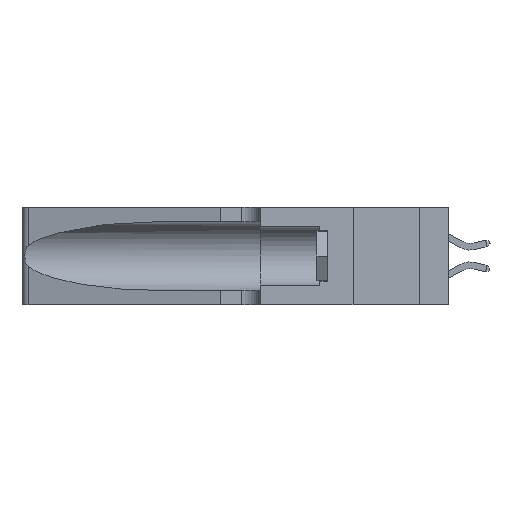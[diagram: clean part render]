
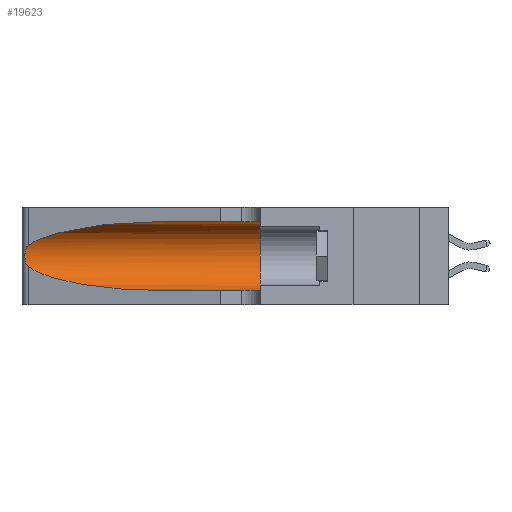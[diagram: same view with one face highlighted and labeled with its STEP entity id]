
A CAD part, left-side view. The second image highlights one B-rep face of the part: STEP entity #19623.
In plain terms, the highlighted cylindrical face has radius 3.308 mm (diameter 6.617 mm), a partial arc.
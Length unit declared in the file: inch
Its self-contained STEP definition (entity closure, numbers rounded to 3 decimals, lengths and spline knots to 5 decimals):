
#348 = EDGE_CURVE ( 'NONE', #20561, #9928, #9784, .T. ) ;
#477 = VERTEX_POINT ( 'NONE', #13632 ) ;
#497 = CARTESIAN_POINT ( 'NONE',  ( 0.25639, 1.23184, 0.21858 ) ) ;
#596 = DIRECTION ( 'NONE',  ( 0., 0., -1. ) ) ;
#694 = CARTESIAN_POINT ( 'NONE',  ( 0.1305, 0.72297, 0.31525 ) ) ;
#824 = CARTESIAN_POINT ( 'NONE',  ( 0.18966, 0.96281, 0.31525 ) ) ;
#1361 = CARTESIAN_POINT ( 'NONE',  ( 0.1305, 0.72297, 0.05475 ) ) ;
#1520 = CARTESIAN_POINT ( 'NONE',  ( 0.1305, 0.35, 0.05475 ) ) ;
#2295 = CARTESIAN_POINT ( 'NONE',  ( 0.25854, 1.2359, 0.20912 ) ) ;
#2627 = CARTESIAN_POINT ( 'NONE',  ( 0.25487, 1.22718, 0.22369 ) ) ;
#2649 =( BOUNDED_CURVE ( )  B_SPLINE_CURVE ( 3, ( #12767, #824, #5948, #2627 ),
 .UNSPECIFIED., .F., .F. ) 
 B_SPLINE_CURVE_WITH_KNOTS ( ( 4, 4 ),
 ( 1.5708, 2.84003 ),
 .UNSPECIFIED. ) 
 CURVE ( )  GEOMETRIC_REPRESENTATION_ITEM ( )  RATIONAL_B_SPLINE_CURVE ( ( 1., 0.87, 0.87, 1. ) ) 
 REPRESENTATION_ITEM ( '' )  );
#2692 = EDGE_CURVE ( 'NONE', #17961, #15681, #2649, .T. ) ;
#4013 = CARTESIAN_POINT ( 'NONE',  ( 0.26075, 1.23896, 0.19203 ) ) ;
#4035 = CARTESIAN_POINT ( 'NONE',  ( 0.25487, 1.22718, 0.14631 ) ) ;
#4983 =( BOUNDED_CURVE ( )  B_SPLINE_CURVE ( 3, ( #10450, #20434, #18830, #8816 ),
 .UNSPECIFIED., .F., .F. ) 
 B_SPLINE_CURVE_WITH_KNOTS ( ( 4, 4 ),
 ( 3.44316, 4.71239 ),
 .UNSPECIFIED. ) 
 CURVE ( )  GEOMETRIC_REPRESENTATION_ITEM ( )  RATIONAL_B_SPLINE_CURVE ( ( 1., 0.87, 0.87, 1. ) ) 
 REPRESENTATION_ITEM ( '' )  );
#5169 = CARTESIAN_POINT ( 'NONE',  ( 0.1305, 1.61858, 0.185 ) ) ;
#5713 = CARTESIAN_POINT ( 'NONE',  ( 0.26017, 1.23833, 0.17102 ) ) ;
#5948 = CARTESIAN_POINT ( 'NONE',  ( 0.2373, 1.15595, 0.28018 ) ) ;
#6148 = ORIENTED_EDGE ( 'NONE', *, *, #12229, .T. ) ;
#6439 = B_SPLINE_CURVE_WITH_KNOTS ( 'NONE', 3,
 ( #7318, #8997, #497, #12452, #2295, #14146, #4013, #15793, #5713, #17450, #7391, #19094, #9061, #20764 ),
 .UNSPECIFIED., .F., .F.,
 ( 4, 2, 2, 2, 2, 2, 4 ),
 ( 0., 0.00027, 0.00053, 0.00107, 0.0016, 0.00187, 0.00214 ),
 .UNSPECIFIED. ) ;
#7070 = DIRECTION ( 'NONE',  ( 0., -1., 0. ) ) ;
#7318 = CARTESIAN_POINT ( 'NONE',  ( 0.25487, 1.22718, 0.22369 ) ) ;
#7391 = CARTESIAN_POINT ( 'NONE',  ( 0.25789, 1.23486, 0.15765 ) ) ;
#7710 = LINE ( 'NONE', #12209, #19467 ) ;
#8169 = CIRCLE ( 'NONE', #14842, 0.13025 ) ;
#8256 = AXIS2_PLACEMENT_3D ( 'NONE', #5169, #10254, #596 ) ;
#8816 = CARTESIAN_POINT ( 'NONE',  ( 0.1305, 0.72297, 0.05475 ) ) ;
#8997 = CARTESIAN_POINT ( 'NONE',  ( 0.25555, 1.22994, 0.2215 ) ) ;
#9061 = CARTESIAN_POINT ( 'NONE',  ( 0.25555, 1.22993, 0.14849 ) ) ;
#9579 = VERTEX_POINT ( 'NONE', #4035 ) ;
#9784 = LINE ( 'NONE', #16242, #18178 ) ;
#9842 = DIRECTION ( 'NONE',  ( 0., 1., 0. ) ) ;
#9928 = VERTEX_POINT ( 'NONE', #1520 ) ;
#10254 = DIRECTION ( 'NONE',  ( 0., -1., 0. ) ) ;
#10450 = CARTESIAN_POINT ( 'NONE',  ( 0.25487, 1.22718, 0.14631 ) ) ;
#12209 = CARTESIAN_POINT ( 'NONE',  ( 0.1305, 1.61858, 0.31525 ) ) ;
#12229 = EDGE_CURVE ( 'NONE', #15681, #9579, #6439, .T. ) ;
#12452 = CARTESIAN_POINT ( 'NONE',  ( 0.25787, 1.23484, 0.2124 ) ) ;
#12767 = CARTESIAN_POINT ( 'NONE',  ( 0.1305, 0.72297, 0.31525 ) ) ;
#13197 = EDGE_CURVE ( 'NONE', #477, #9928, #8169, .T. ) ;
#13479 = FACE_OUTER_BOUND ( 'NONE', #16182, .T. ) ;
#13497 = EDGE_CURVE ( 'NONE', #9579, #20561, #4983, .T. ) ;
#13632 = CARTESIAN_POINT ( 'NONE',  ( 0.1305, 0.35, 0.31525 ) ) ;
#14146 = CARTESIAN_POINT ( 'NONE',  ( 0.26018, 1.23835, 0.19895 ) ) ;
#14842 = AXIS2_PLACEMENT_3D ( 'NONE', #19849, #9842, #21498 ) ;
#15394 = ORIENTED_EDGE ( 'NONE', *, *, #13197, .F. ) ;
#15681 = VERTEX_POINT ( 'NONE', #20165 ) ;
#15793 = CARTESIAN_POINT ( 'NONE',  ( 0.26075, 1.23896, 0.178 ) ) ;
#16182 = EDGE_LOOP ( 'NONE', ( #18990, #6148, #19497, #16521, #15394, #21078 ) ) ;
#16242 = CARTESIAN_POINT ( 'NONE',  ( 0.1305, 1.61858, 0.05475 ) ) ;
#16521 = ORIENTED_EDGE ( 'NONE', *, *, #348, .T. ) ;
#17204 = DIRECTION ( 'NONE',  ( 0., -1., 0. ) ) ;
#17450 = CARTESIAN_POINT ( 'NONE',  ( 0.25856, 1.23593, 0.16098 ) ) ;
#17784 = EDGE_CURVE ( 'NONE', #17961, #477, #7710, .T. ) ;
#17961 = VERTEX_POINT ( 'NONE', #694 ) ;
#18178 = VECTOR ( 'NONE', #17204, 39.37008 ) ;
#18830 = CARTESIAN_POINT ( 'NONE',  ( 0.18966, 0.96281, 0.05475 ) ) ;
#18990 = ORIENTED_EDGE ( 'NONE', *, *, #2692, .T. ) ;
#19094 = CARTESIAN_POINT ( 'NONE',  ( 0.25639, 1.23186, 0.15144 ) ) ;
#19467 = VECTOR ( 'NONE', #7070, 39.37008 ) ;
#19497 = ORIENTED_EDGE ( 'NONE', *, *, #13497, .T. ) ;
#19623 = ADVANCED_FACE ( 'NONE', ( #13479 ), #21712, .F. ) ;
#19849 = CARTESIAN_POINT ( 'NONE',  ( 0.1305, 0.35, 0.185 ) ) ;
#20165 = CARTESIAN_POINT ( 'NONE',  ( 0.25487, 1.22718, 0.22369 ) ) ;
#20434 = CARTESIAN_POINT ( 'NONE',  ( 0.2373, 1.15595, 0.08982 ) ) ;
#20561 = VERTEX_POINT ( 'NONE', #1361 ) ;
#20764 = CARTESIAN_POINT ( 'NONE',  ( 0.25487, 1.22718, 0.14631 ) ) ;
#21078 = ORIENTED_EDGE ( 'NONE', *, *, #17784, .F. ) ;
#21498 = DIRECTION ( 'NONE',  ( 0., 0., 1. ) ) ;
#21712 = CYLINDRICAL_SURFACE ( 'NONE', #8256, 0.13025 ) ;
